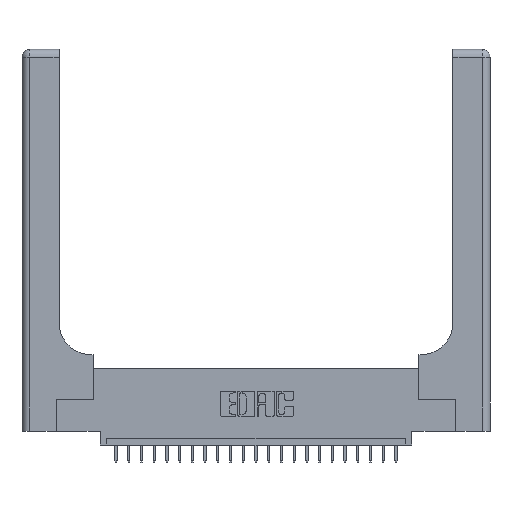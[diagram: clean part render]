
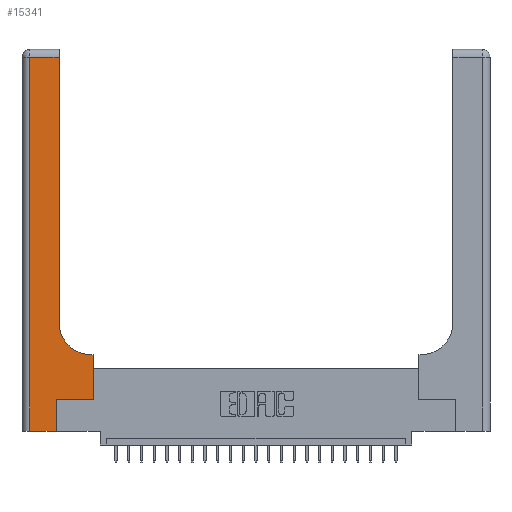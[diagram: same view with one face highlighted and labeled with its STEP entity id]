
A CAD part, top view. The second image highlights one B-rep face of the part: STEP entity #15341.
In plain terms, the highlighted planar face has unit normal (0, 0, 1).
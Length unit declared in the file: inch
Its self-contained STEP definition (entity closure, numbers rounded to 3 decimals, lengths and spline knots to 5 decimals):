
#778 = CARTESIAN_POINT ( 'NONE',  ( 0.5415, 0.6, 0.37 ) ) ;
#885 = DIRECTION ( 'NONE',  ( 0., 0., -1. ) ) ;
#2608 = ORIENTED_EDGE ( 'NONE', *, *, #7076, .T. ) ;
#2918 = DIRECTION ( 'NONE',  ( 0., 1., 0. ) ) ;
#3133 = CARTESIAN_POINT ( 'NONE',  ( 0.269, 0.25, 0.37 ) ) ;
#3180 = EDGE_CURVE ( 'NONE', #6722, #25155, #5642, .T. ) ;
#4470 = VERTEX_POINT ( 'NONE', #6133 ) ;
#4739 = CARTESIAN_POINT ( 'NONE',  ( 0.2915, 0.85, 0.37 ) ) ;
#4920 = DIRECTION ( 'NONE',  ( 1., 0., 0. ) ) ;
#5003 = DIRECTION ( 'NONE',  ( 0., 1., 0. ) ) ;
#5070 = VECTOR ( 'NONE', #2918, 39.37008 ) ;
#5126 = VECTOR ( 'NONE', #5003, 39.37008 ) ;
#5176 = VERTEX_POINT ( 'NONE', #11306 ) ;
#5642 = LINE ( 'NONE', #3133, #21311 ) ;
#5982 = DIRECTION ( 'NONE',  ( -1., 0., 0. ) ) ;
#6133 = CARTESIAN_POINT ( 'NONE',  ( 0.5585, 0.6, 0.37 ) ) ;
#6298 = DIRECTION ( 'NONE',  ( -1., 0., 0. ) ) ;
#6335 = VECTOR ( 'NONE', #22454, 39.37008 ) ;
#6396 = VECTOR ( 'NONE', #6298, 39.37008 ) ;
#6538 = ORIENTED_EDGE ( 'NONE', *, *, #18001, .T. ) ;
#6722 = VERTEX_POINT ( 'NONE', #9931 ) ;
#7076 = EDGE_CURVE ( 'NONE', #10705, #18445, #14250, .T. ) ;
#7471 = ORIENTED_EDGE ( 'NONE', *, *, #19878, .T. ) ;
#7657 = AXIS2_PLACEMENT_3D ( 'NONE', #23527, #15958, #5982 ) ;
#7734 = CARTESIAN_POINT ( 'NONE',  ( 0., 0., 0.37 ) ) ;
#8168 = PLANE ( 'NONE',  #7657 ) ;
#8449 = CARTESIAN_POINT ( 'NONE',  ( 0.5585, 0.25, 0.37 ) ) ;
#8784 = LINE ( 'NONE', #20522, #6335 ) ;
#8884 = CARTESIAN_POINT ( 'NONE',  ( 0.5585, 0.25, 0.37 ) ) ;
#9039 = LINE ( 'NONE', #7734, #9786 ) ;
#9311 = LINE ( 'NONE', #17103, #21885 ) ;
#9752 = ORIENTED_EDGE ( 'NONE', *, *, #20252, .T. ) ;
#9786 = VECTOR ( 'NONE', #13271, 39.37008 ) ;
#9931 = CARTESIAN_POINT ( 'NONE',  ( 0.269, 0.25, 0.37 ) ) ;
#10356 = ORIENTED_EDGE ( 'NONE', *, *, #21742, .T. ) ;
#10416 = CARTESIAN_POINT ( 'NONE',  ( 0., 2.94, 0.37 ) ) ;
#10650 = CARTESIAN_POINT ( 'NONE',  ( 0.5415, 0.85, 0.37 ) ) ;
#10652 = ORIENTED_EDGE ( 'NONE', *, *, #10670, .T. ) ;
#10670 = EDGE_CURVE ( 'NONE', #25155, #4470, #24311, .T. ) ;
#10705 = VERTEX_POINT ( 'NONE', #16251 ) ;
#10950 = CARTESIAN_POINT ( 'NONE',  ( 0.2915, 3., 0.37 ) ) ;
#10960 = CIRCLE ( 'NONE', #25204, 0.25 ) ;
#11306 = CARTESIAN_POINT ( 'NONE',  ( 0.06, 0., 0.37 ) ) ;
#11632 = DIRECTION ( 'NONE',  ( 0., 1., 0. ) ) ;
#12282 = VERTEX_POINT ( 'NONE', #778 ) ;
#12741 = DIRECTION ( 'NONE',  ( -1., 0., 0. ) ) ;
#13271 = DIRECTION ( 'NONE',  ( 1., 0., 0. ) ) ;
#13493 = EDGE_CURVE ( 'NONE', #24604, #10705, #24478, .T. ) ;
#14250 = LINE ( 'NONE', #10416, #23347 ) ;
#15341 = ADVANCED_FACE ( 'NONE', ( #17500 ), #8168, .F. ) ;
#15958 = DIRECTION ( 'NONE',  ( 0., 0., -1. ) ) ;
#16251 = CARTESIAN_POINT ( 'NONE',  ( 0.2915, 2.94, 0.37 ) ) ;
#16501 = DIRECTION ( 'NONE',  ( 1., 0., 0. ) ) ;
#17103 = CARTESIAN_POINT ( 'NONE',  ( 0.269, 0., 0.37 ) ) ;
#17158 = CARTESIAN_POINT ( 'NONE',  ( 0.06, 2.94, 0.37 ) ) ;
#17500 = FACE_OUTER_BOUND ( 'NONE', #20877, .T. ) ;
#17522 = ORIENTED_EDGE ( 'NONE', *, *, #3180, .T. ) ;
#17909 = ORIENTED_EDGE ( 'NONE', *, *, #21592, .T. ) ;
#17949 = LINE ( 'NONE', #18467, #6396 ) ;
#18001 = EDGE_CURVE ( 'NONE', #5176, #18102, #9039, .T. ) ;
#18102 = VERTEX_POINT ( 'NONE', #23215 ) ;
#18445 = VERTEX_POINT ( 'NONE', #17158 ) ;
#18467 = CARTESIAN_POINT ( 'NONE',  ( 0.2915, 0.6, 0.37 ) ) ;
#19878 = EDGE_CURVE ( 'NONE', #18102, #6722, #9311, .T. ) ;
#20252 = EDGE_CURVE ( 'NONE', #18445, #5176, #8784, .T. ) ;
#20522 = CARTESIAN_POINT ( 'NONE',  ( 0.06, 3., 0.37 ) ) ;
#20877 = EDGE_LOOP ( 'NONE', ( #24885, #2608, #9752, #6538, #7471, #17522, #10652, #10356, #17909 ) ) ;
#21311 = VECTOR ( 'NONE', #4920, 39.37008 ) ;
#21592 = EDGE_CURVE ( 'NONE', #12282, #24604, #10960, .T. ) ;
#21742 = EDGE_CURVE ( 'NONE', #4470, #12282, #17949, .T. ) ;
#21885 = VECTOR ( 'NONE', #11632, 39.37008 ) ;
#22454 = DIRECTION ( 'NONE',  ( 0., -1., 0. ) ) ;
#23215 = CARTESIAN_POINT ( 'NONE',  ( 0.269, 0., 0.37 ) ) ;
#23347 = VECTOR ( 'NONE', #12741, 39.37008 ) ;
#23527 = CARTESIAN_POINT ( 'NONE',  ( 0., 3., 0.37 ) ) ;
#24311 = LINE ( 'NONE', #8449, #5070 ) ;
#24478 = LINE ( 'NONE', #10950, #5126 ) ;
#24604 = VERTEX_POINT ( 'NONE', #4739 ) ;
#24885 = ORIENTED_EDGE ( 'NONE', *, *, #13493, .T. ) ;
#25155 = VERTEX_POINT ( 'NONE', #8884 ) ;
#25204 = AXIS2_PLACEMENT_3D ( 'NONE', #10650, #885, #16501 ) ;
